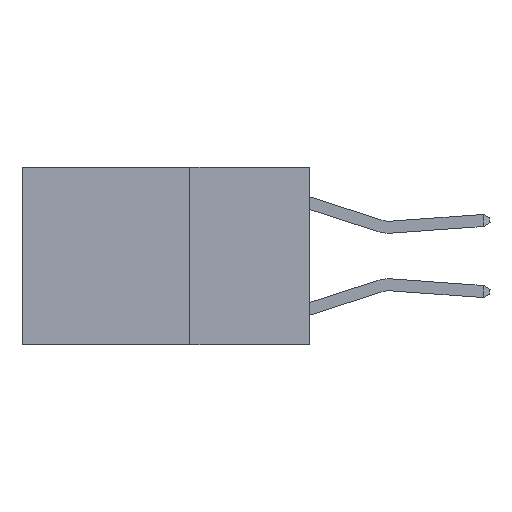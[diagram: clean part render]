
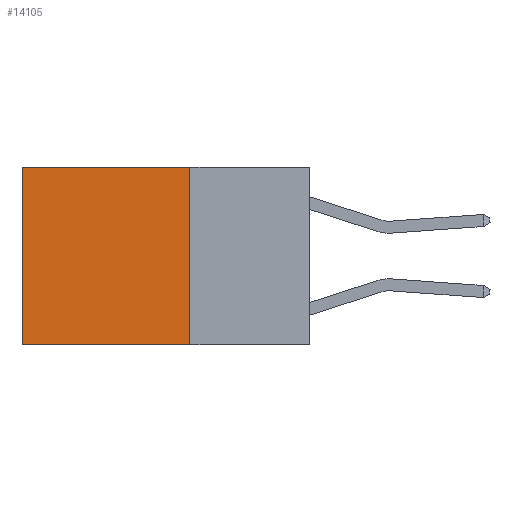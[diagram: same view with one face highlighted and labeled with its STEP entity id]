
A CAD part, left-side view. The second image highlights one B-rep face of the part: STEP entity #14105.
In plain terms, the highlighted planar face has unit normal (-1, 0, 0).
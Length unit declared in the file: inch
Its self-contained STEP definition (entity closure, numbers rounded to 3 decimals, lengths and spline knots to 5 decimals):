
#135 = AXIS2_PLACEMENT_3D ( 'NONE', #12567, #10254, #3092 ) ;
#990 = EDGE_LOOP ( 'NONE', ( #2686, #4825, #1622, #14993 ) ) ;
#1191 = DIRECTION ( 'NONE',  ( 0., 1., 0. ) ) ;
#1340 = LINE ( 'NONE', #3883, #1501 ) ;
#1501 = VECTOR ( 'NONE', #6080, 39.37008 ) ;
#1622 = ORIENTED_EDGE ( 'NONE', *, *, #10858, .F. ) ;
#2686 = ORIENTED_EDGE ( 'NONE', *, *, #10508, .T. ) ;
#3092 = DIRECTION ( 'NONE',  ( 0., 0., -1. ) ) ;
#3363 = LINE ( 'NONE', #14035, #5242 ) ;
#3867 = CARTESIAN_POINT ( 'NONE',  ( 0.2625, 0.25, 0. ) ) ;
#3883 = CARTESIAN_POINT ( 'NONE',  ( 0.2625, 0.25, 0. ) ) ;
#4705 = DIRECTION ( 'NONE',  ( 0., 0., -1. ) ) ;
#4825 = ORIENTED_EDGE ( 'NONE', *, *, #9188, .F. ) ;
#5157 = DIRECTION ( 'NONE',  ( 0., 0., -1. ) ) ;
#5242 = VECTOR ( 'NONE', #4705, 39.37008 ) ;
#5588 = PLANE ( 'NONE',  #135 ) ;
#6080 = DIRECTION ( 'NONE',  ( 0., 1., 0. ) ) ;
#6963 = VECTOR ( 'NONE', #5157, 39.37008 ) ;
#7143 = LINE ( 'NONE', #12919, #8878 ) ;
#7680 = CARTESIAN_POINT ( 'NONE',  ( 0.2625, 0.25, 0. ) ) ;
#7728 = FACE_OUTER_BOUND ( 'NONE', #990, .T. ) ;
#8873 = CARTESIAN_POINT ( 'NONE',  ( 0.2625, 0.25, -0.37 ) ) ;
#8878 = VECTOR ( 'NONE', #1191, 39.37008 ) ;
#8905 = LINE ( 'NONE', #7680, #6963 ) ;
#9188 = EDGE_CURVE ( 'NONE', #14072, #10455, #7143, .T. ) ;
#9404 = EDGE_CURVE ( 'NONE', #9780, #14738, #1340, .T. ) ;
#9780 = VERTEX_POINT ( 'NONE', #3867 ) ;
#10254 = DIRECTION ( 'NONE',  ( 1., 0., 0. ) ) ;
#10455 = VERTEX_POINT ( 'NONE', #14728 ) ;
#10508 = EDGE_CURVE ( 'NONE', #14738, #10455, #3363, .T. ) ;
#10858 = EDGE_CURVE ( 'NONE', #9780, #14072, #8905, .T. ) ;
#11699 = CARTESIAN_POINT ( 'NONE',  ( 0.2625, 0.6, 0. ) ) ;
#12567 = CARTESIAN_POINT ( 'NONE',  ( 0.2625, 0.25, 0. ) ) ;
#12919 = CARTESIAN_POINT ( 'NONE',  ( 0.2625, 0.25, -0.37 ) ) ;
#14035 = CARTESIAN_POINT ( 'NONE',  ( 0.2625, 0.6, 0. ) ) ;
#14072 = VERTEX_POINT ( 'NONE', #8873 ) ;
#14105 = ADVANCED_FACE ( 'NONE', ( #7728 ), #5588, .F. ) ;
#14728 = CARTESIAN_POINT ( 'NONE',  ( 0.2625, 0.6, -0.37 ) ) ;
#14738 = VERTEX_POINT ( 'NONE', #11699 ) ;
#14993 = ORIENTED_EDGE ( 'NONE', *, *, #9404, .T. ) ;
